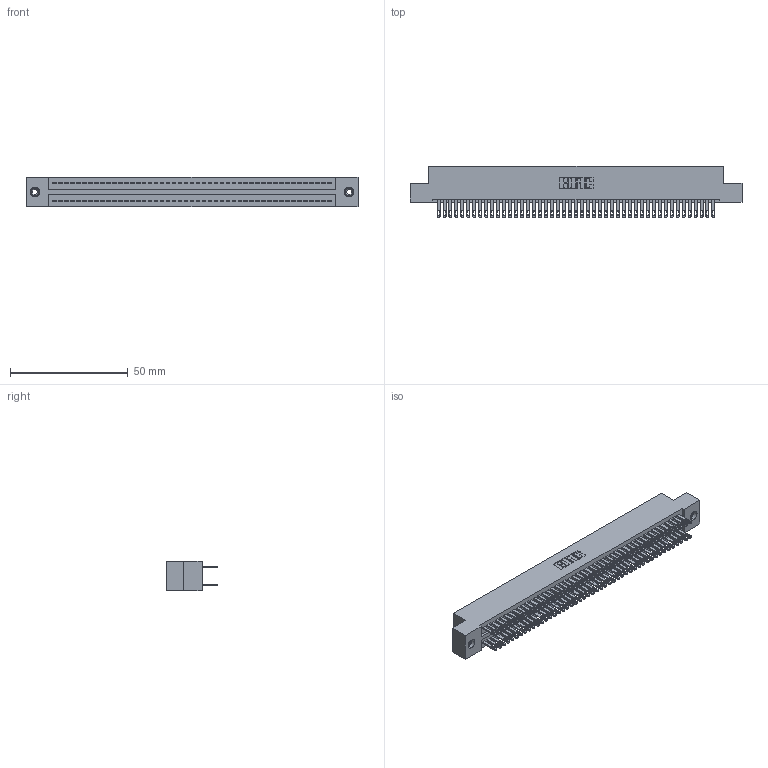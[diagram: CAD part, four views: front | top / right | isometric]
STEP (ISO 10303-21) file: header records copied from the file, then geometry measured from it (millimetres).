
FILE_DESCRIPTION (( 'STEP AP203' ), '1' );
FILE_NAME ('325-094-500-208.STEP', '2020-02-25T05:58:25', ( '' ), ( '' ), 'SwSTEP 2.0', 'SolidWorks 2016', '' );
FILE_SCHEMA (( 'CONFIG_CONTROL_DESIGN' ));
Length unit declared in the file: inch
Products named in the file (4): 345-250-001_345-250-003-102; 325-094-500-208; 325-292-001_325-293-100; 325 Part_TI
Assembly tree (97 placements, depth 2):
  325-094-500-208
    325 Part_TI
    325-292-001_325-293-100  x94
    345-250-001_345-250-003-102  x2
Bounding box: 141.1 x 21.84 x 12.45 mm (x, y, z)
Volume: 18540.6 mm3; surface area: 23556.1 mm2
Topology: 97 solids, 97 shells, 4686 faces, 14265 edges, 9502 vertices
Faces by surface type: plane 2922, cylinder 1748, cone 12, torus 4
Entity records: 30706 total; most frequent: CARTESIAN_POINT 5065, ORIENTED_EDGE 4994, DIRECTION 4351, EDGE_CURVE 2497, LINE 2345, VECTOR 2345, VERTEX_POINT 1660, AXIS2_PLACEMENT_3D 1003
